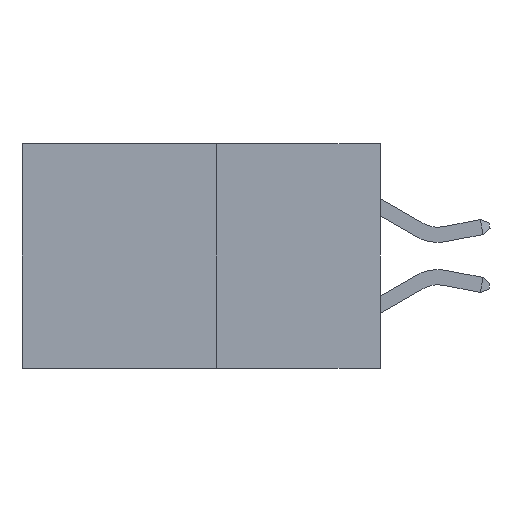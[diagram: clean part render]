
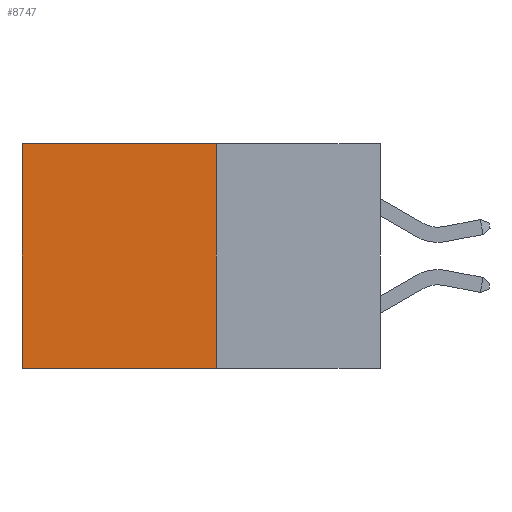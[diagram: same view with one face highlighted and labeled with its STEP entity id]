
A CAD part, left-side view. The second image highlights one B-rep face of the part: STEP entity #8747.
In plain terms, the highlighted planar face has unit normal (-1, 0, 0).
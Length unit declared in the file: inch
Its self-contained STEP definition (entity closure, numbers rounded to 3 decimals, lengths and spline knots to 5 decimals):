
#373 = VECTOR ( 'NONE', #15314, 39.37008 ) ;
#1375 = EDGE_CURVE ( 'NONE', #13226, #16375, #5704, .T. ) ;
#2170 = CARTESIAN_POINT ( 'NONE',  ( 0.277, 0.59, -0.37 ) ) ;
#2496 = DIRECTION ( 'NONE',  ( 1., 0., 0. ) ) ;
#2649 = CARTESIAN_POINT ( 'NONE',  ( 0.277, 0.27, 0. ) ) ;
#2755 = VERTEX_POINT ( 'NONE', #11327 ) ;
#3367 = VECTOR ( 'NONE', #13116, 39.37008 ) ;
#4053 = VERTEX_POINT ( 'NONE', #12715 ) ;
#4094 = ORIENTED_EDGE ( 'NONE', *, *, #9250, .F. ) ;
#4120 = CARTESIAN_POINT ( 'NONE',  ( 0.277, 0.59, 0. ) ) ;
#4522 = ORIENTED_EDGE ( 'NONE', *, *, #15254, .T. ) ;
#5704 = LINE ( 'NONE', #11105, #15217 ) ;
#6790 = VECTOR ( 'NONE', #10018, 39.37008 ) ;
#7585 = CARTESIAN_POINT ( 'NONE',  ( 0.277, 0.27, -0.37 ) ) ;
#7630 = ORIENTED_EDGE ( 'NONE', *, *, #12201, .F. ) ;
#8693 = CARTESIAN_POINT ( 'NONE',  ( 0.277, 0.27, -0.37 ) ) ;
#8747 = ADVANCED_FACE ( 'NONE', ( #16658 ), #14248, .F. ) ;
#9250 = EDGE_CURVE ( 'NONE', #4053, #16375, #16648, .T. ) ;
#10018 = DIRECTION ( 'NONE',  ( 0., 1., 0. ) ) ;
#10435 = CARTESIAN_POINT ( 'NONE',  ( 0.277, 0.27, -0.37 ) ) ;
#10842 = LINE ( 'NONE', #2649, #3367 ) ;
#11105 = CARTESIAN_POINT ( 'NONE',  ( 0.277, 0.59, -0.37 ) ) ;
#11327 = CARTESIAN_POINT ( 'NONE',  ( 0.277, 0.27, 0. ) ) ;
#11680 = AXIS2_PLACEMENT_3D ( 'NONE', #10435, #2496, #11732 ) ;
#11732 = DIRECTION ( 'NONE',  ( 0., 0., -1. ) ) ;
#11877 = DIRECTION ( 'NONE',  ( 0., 0., -1. ) ) ;
#12201 = EDGE_CURVE ( 'NONE', #2755, #4053, #14326, .T. ) ;
#12715 = CARTESIAN_POINT ( 'NONE',  ( 0.277, 0.27, -0.37 ) ) ;
#13116 = DIRECTION ( 'NONE',  ( 0., 1., 0. ) ) ;
#13226 = VERTEX_POINT ( 'NONE', #4120 ) ;
#13239 = EDGE_LOOP ( 'NONE', ( #16659, #4094, #7630, #4522 ) ) ;
#14248 = PLANE ( 'NONE',  #11680 ) ;
#14326 = LINE ( 'NONE', #7585, #373 ) ;
#15217 = VECTOR ( 'NONE', #11877, 39.37008 ) ;
#15254 = EDGE_CURVE ( 'NONE', #2755, #13226, #10842, .T. ) ;
#15314 = DIRECTION ( 'NONE',  ( 0., 0., -1. ) ) ;
#16375 = VERTEX_POINT ( 'NONE', #2170 ) ;
#16648 = LINE ( 'NONE', #8693, #6790 ) ;
#16658 = FACE_OUTER_BOUND ( 'NONE', #13239, .T. ) ;
#16659 = ORIENTED_EDGE ( 'NONE', *, *, #1375, .T. ) ;
